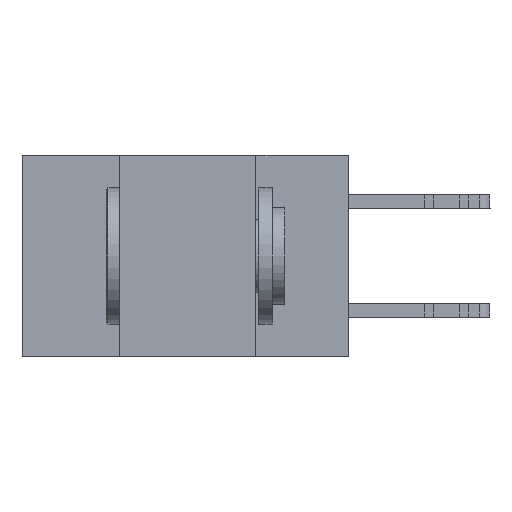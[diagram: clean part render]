
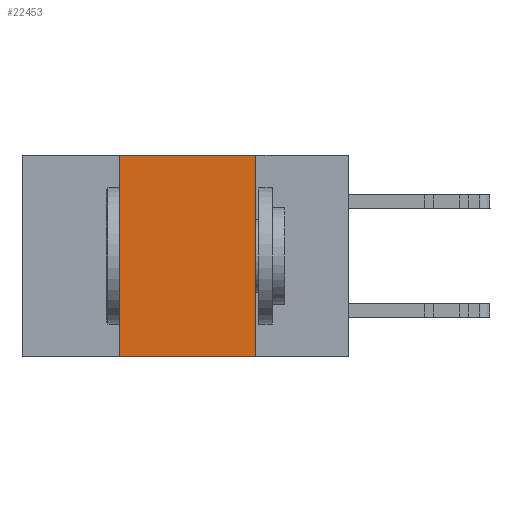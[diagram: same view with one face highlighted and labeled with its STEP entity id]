
A CAD part, left-side view. The second image highlights one B-rep face of the part: STEP entity #22453.
In plain terms, the highlighted planar face has unit normal (-1, 0, 0).
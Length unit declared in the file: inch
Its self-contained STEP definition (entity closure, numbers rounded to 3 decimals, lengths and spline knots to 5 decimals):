
#1628 = DIRECTION ( 'NONE',  ( 0., -1., 0. ) ) ;
#1709 = LINE ( 'NONE', #1993, #7912 ) ;
#1993 = CARTESIAN_POINT ( 'NONE',  ( 0., 0.17, 0. ) ) ;
#2626 = DIRECTION ( 'NONE',  ( 1., 0., 0. ) ) ;
#2818 = VERTEX_POINT ( 'NONE', #16100 ) ;
#3155 = EDGE_LOOP ( 'NONE', ( #26742, #22038, #28142, #25668 ) ) ;
#3610 = VECTOR ( 'NONE', #1628, 39.37008 ) ;
#4322 = DIRECTION ( 'NONE',  ( 0., 0., -1. ) ) ;
#4393 = VERTEX_POINT ( 'NONE', #11222 ) ;
#5492 = VECTOR ( 'NONE', #7235, 39.37008 ) ;
#7235 = DIRECTION ( 'NONE',  ( 0., 0., 1. ) ) ;
#7521 = DIRECTION ( 'NONE',  ( 0., -1., 0. ) ) ;
#7912 = VECTOR ( 'NONE', #4322, 39.37008 ) ;
#10387 = FACE_OUTER_BOUND ( 'NONE', #3155, .T. ) ;
#10598 = LINE ( 'NONE', #17952, #3610 ) ;
#10625 = CARTESIAN_POINT ( 'NONE',  ( 0., 0.42, -0.37 ) ) ;
#11222 = CARTESIAN_POINT ( 'NONE',  ( 0., 0.42, 0. ) ) ;
#11696 = VERTEX_POINT ( 'NONE', #16527 ) ;
#14252 = PLANE ( 'NONE',  #26067 ) ;
#14471 = CARTESIAN_POINT ( 'NONE',  ( 0., 0.6, 0. ) ) ;
#16100 = CARTESIAN_POINT ( 'NONE',  ( 0., 0.17, -0.37 ) ) ;
#16527 = CARTESIAN_POINT ( 'NONE',  ( 0., 0.17, 0. ) ) ;
#16530 = CARTESIAN_POINT ( 'NONE',  ( 0., 0.42, 0. ) ) ;
#16575 = CARTESIAN_POINT ( 'NONE',  ( 0., 0.6, 0. ) ) ;
#17155 = LINE ( 'NONE', #16530, #5492 ) ;
#17952 = CARTESIAN_POINT ( 'NONE',  ( 0., 0.6, -0.37 ) ) ;
#18921 = DIRECTION ( 'NONE',  ( 0., 0., -1. ) ) ;
#19751 = EDGE_CURVE ( 'NONE', #24142, #2818, #10598, .T. ) ;
#20615 = EDGE_CURVE ( 'NONE', #11696, #2818, #1709, .T. ) ;
#22038 = ORIENTED_EDGE ( 'NONE', *, *, #24887, .F. ) ;
#22453 = ADVANCED_FACE ( 'NONE', ( #10387 ), #14252, .F. ) ;
#24142 = VERTEX_POINT ( 'NONE', #10625 ) ;
#24240 = EDGE_CURVE ( 'NONE', #24142, #4393, #17155, .T. ) ;
#24394 = LINE ( 'NONE', #14471, #29774 ) ;
#24887 = EDGE_CURVE ( 'NONE', #4393, #11696, #24394, .T. ) ;
#25668 = ORIENTED_EDGE ( 'NONE', *, *, #19751, .T. ) ;
#26067 = AXIS2_PLACEMENT_3D ( 'NONE', #16575, #2626, #18921 ) ;
#26742 = ORIENTED_EDGE ( 'NONE', *, *, #20615, .F. ) ;
#28142 = ORIENTED_EDGE ( 'NONE', *, *, #24240, .F. ) ;
#29774 = VECTOR ( 'NONE', #7521, 39.37008 ) ;
